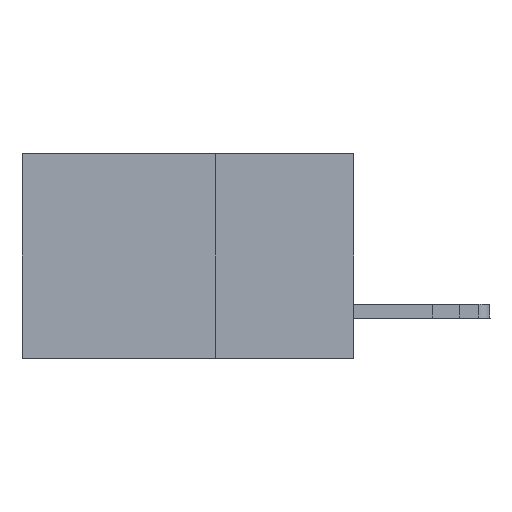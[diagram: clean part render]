
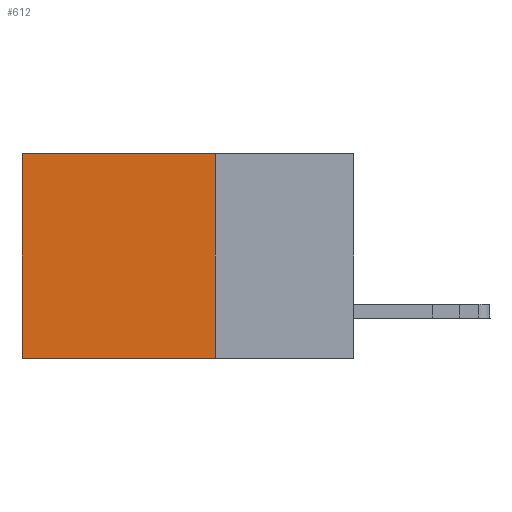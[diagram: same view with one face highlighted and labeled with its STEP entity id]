
A CAD part, left-side view. The second image highlights one B-rep face of the part: STEP entity #612.
In plain terms, the highlighted planar face has unit normal (-1, 0, 0).
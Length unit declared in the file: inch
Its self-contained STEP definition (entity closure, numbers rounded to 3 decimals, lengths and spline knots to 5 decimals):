
#145 = LINE ( 'NONE', #9098, #24871 ) ;
#201 = VERTEX_POINT ( 'NONE', #13024 ) ;
#425 = EDGE_LOOP ( 'NONE', ( #21609, #18045, #29475, #13067 ) ) ;
#612 = ADVANCED_FACE ( 'NONE', ( #12086 ), #6585, .F. ) ;
#1555 = CARTESIAN_POINT ( 'NONE',  ( 0.2875, 0.6, 0. ) ) ;
#4391 = DIRECTION ( 'NONE',  ( 0., 0., -1. ) ) ;
#4895 = VECTOR ( 'NONE', #18969, 39.37008 ) ;
#6321 = AXIS2_PLACEMENT_3D ( 'NONE', #25450, #26322, #13427 ) ;
#6585 = PLANE ( 'NONE',  #6321 ) ;
#7086 = CARTESIAN_POINT ( 'NONE',  ( 0.2875, 0.25, 0. ) ) ;
#9098 = CARTESIAN_POINT ( 'NONE',  ( 0.2875, 0.25, 0. ) ) ;
#9509 = DIRECTION ( 'NONE',  ( 0., 1., 0. ) ) ;
#10040 = EDGE_CURVE ( 'NONE', #24248, #11340, #22724, .T. ) ;
#10316 = LINE ( 'NONE', #7086, #22269 ) ;
#11340 = VERTEX_POINT ( 'NONE', #27803 ) ;
#12086 = FACE_OUTER_BOUND ( 'NONE', #425, .T. ) ;
#12279 = EDGE_CURVE ( 'NONE', #18642, #201, #145, .T. ) ;
#13024 = CARTESIAN_POINT ( 'NONE',  ( 0.2875, 0.25, -0.37 ) ) ;
#13067 = ORIENTED_EDGE ( 'NONE', *, *, #18385, .T. ) ;
#13427 = DIRECTION ( 'NONE',  ( 0., 0., -1. ) ) ;
#17558 = CARTESIAN_POINT ( 'NONE',  ( 0.2875, 0.25, 0. ) ) ;
#18045 = ORIENTED_EDGE ( 'NONE', *, *, #25297, .F. ) ;
#18385 = EDGE_CURVE ( 'NONE', #18642, #24248, #10316, .T. ) ;
#18642 = VERTEX_POINT ( 'NONE', #17558 ) ;
#18969 = DIRECTION ( 'NONE',  ( 0., 1., 0. ) ) ;
#21609 = ORIENTED_EDGE ( 'NONE', *, *, #10040, .T. ) ;
#22269 = VECTOR ( 'NONE', #9509, 39.37008 ) ;
#22724 = LINE ( 'NONE', #25292, #28280 ) ;
#23980 = LINE ( 'NONE', #30809, #4895 ) ;
#24248 = VERTEX_POINT ( 'NONE', #1555 ) ;
#24871 = VECTOR ( 'NONE', #4391, 39.37008 ) ;
#25292 = CARTESIAN_POINT ( 'NONE',  ( 0.2875, 0.6, 0. ) ) ;
#25297 = EDGE_CURVE ( 'NONE', #201, #11340, #23980, .T. ) ;
#25450 = CARTESIAN_POINT ( 'NONE',  ( 0.2875, 0.25, 0. ) ) ;
#26322 = DIRECTION ( 'NONE',  ( 1., 0., 0. ) ) ;
#27766 = DIRECTION ( 'NONE',  ( 0., 0., -1. ) ) ;
#27803 = CARTESIAN_POINT ( 'NONE',  ( 0.2875, 0.6, -0.37 ) ) ;
#28280 = VECTOR ( 'NONE', #27766, 39.37008 ) ;
#29475 = ORIENTED_EDGE ( 'NONE', *, *, #12279, .F. ) ;
#30809 = CARTESIAN_POINT ( 'NONE',  ( 0.2875, 0.25, -0.37 ) ) ;
